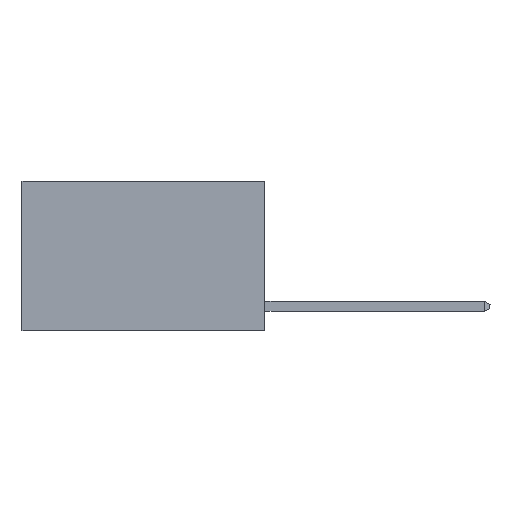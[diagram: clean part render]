
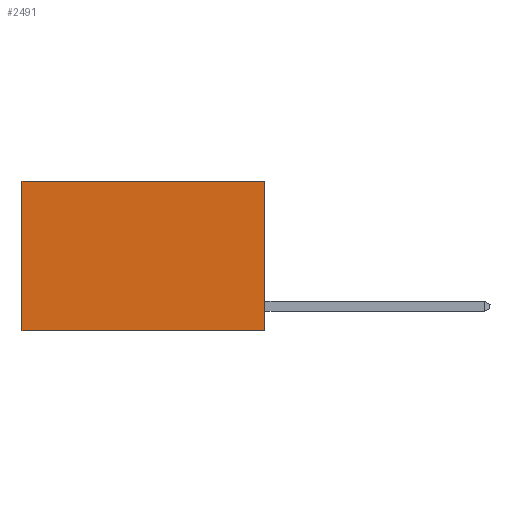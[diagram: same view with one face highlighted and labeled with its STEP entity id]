
A CAD part, left-side view. The second image highlights one B-rep face of the part: STEP entity #2491.
In plain terms, the highlighted planar face has unit normal (-1, 0, 0).
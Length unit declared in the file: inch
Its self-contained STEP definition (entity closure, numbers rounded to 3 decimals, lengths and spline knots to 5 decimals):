
#609 = LINE ( 'NONE', #18968, #20806 ) ;
#1474 = DIRECTION ( 'NONE',  ( 0., 1., 0. ) ) ;
#1680 = CARTESIAN_POINT ( 'NONE',  ( 0.2625, 0., 0. ) ) ;
#2491 = ADVANCED_FACE ( 'NONE', ( #22839 ), #2917, .F. ) ;
#2917 = PLANE ( 'NONE',  #9495 ) ;
#3429 = DIRECTION ( 'NONE',  ( 0., 1., 0. ) ) ;
#3654 = EDGE_LOOP ( 'NONE', ( #15958, #10444, #11100, #16584 ) ) ;
#3700 = LINE ( 'NONE', #19522, #23882 ) ;
#5497 = EDGE_CURVE ( 'NONE', #24234, #17249, #3700, .T. ) ;
#6586 = EDGE_CURVE ( 'NONE', #24062, #14189, #23671, .T. ) ;
#6830 = DIRECTION ( 'NONE',  ( 0., 0., -1. ) ) ;
#7437 = VECTOR ( 'NONE', #11001, 39.37008 ) ;
#9106 = CARTESIAN_POINT ( 'NONE',  ( 0.2625, 0.6, -0.37 ) ) ;
#9495 = AXIS2_PLACEMENT_3D ( 'NONE', #16557, #18535, #6830 ) ;
#9809 = EDGE_CURVE ( 'NONE', #24234, #24062, #609, .T. ) ;
#10444 = ORIENTED_EDGE ( 'NONE', *, *, #11815, .F. ) ;
#11001 = DIRECTION ( 'NONE',  ( 0., 0., -1. ) ) ;
#11100 = ORIENTED_EDGE ( 'NONE', *, *, #5497, .F. ) ;
#11815 = EDGE_CURVE ( 'NONE', #17249, #14189, #13081, .T. ) ;
#13081 = LINE ( 'NONE', #18950, #22899 ) ;
#14189 = VERTEX_POINT ( 'NONE', #9106 ) ;
#15757 = CARTESIAN_POINT ( 'NONE',  ( 0.2625, 0., -0.37 ) ) ;
#15958 = ORIENTED_EDGE ( 'NONE', *, *, #6586, .T. ) ;
#16557 = CARTESIAN_POINT ( 'NONE',  ( 0.2625, 0., 0. ) ) ;
#16584 = ORIENTED_EDGE ( 'NONE', *, *, #9809, .T. ) ;
#17249 = VERTEX_POINT ( 'NONE', #15757 ) ;
#18535 = DIRECTION ( 'NONE',  ( 1., 0., 0. ) ) ;
#18950 = CARTESIAN_POINT ( 'NONE',  ( 0.2625, 0., -0.37 ) ) ;
#18968 = CARTESIAN_POINT ( 'NONE',  ( 0.2625, 0., 0. ) ) ;
#19522 = CARTESIAN_POINT ( 'NONE',  ( 0.2625, 0., 0. ) ) ;
#20806 = VECTOR ( 'NONE', #1474, 39.37008 ) ;
#22728 = CARTESIAN_POINT ( 'NONE',  ( 0.2625, 0.6, 0. ) ) ;
#22839 = FACE_OUTER_BOUND ( 'NONE', #3654, .T. ) ;
#22899 = VECTOR ( 'NONE', #3429, 39.37008 ) ;
#23464 = DIRECTION ( 'NONE',  ( 0., 0., -1. ) ) ;
#23671 = LINE ( 'NONE', #24699, #7437 ) ;
#23882 = VECTOR ( 'NONE', #23464, 39.37008 ) ;
#24062 = VERTEX_POINT ( 'NONE', #22728 ) ;
#24234 = VERTEX_POINT ( 'NONE', #1680 ) ;
#24699 = CARTESIAN_POINT ( 'NONE',  ( 0.2625, 0.6, 0. ) ) ;
